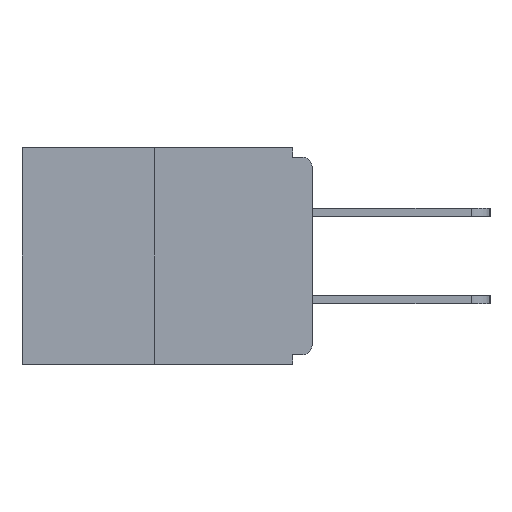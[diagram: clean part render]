
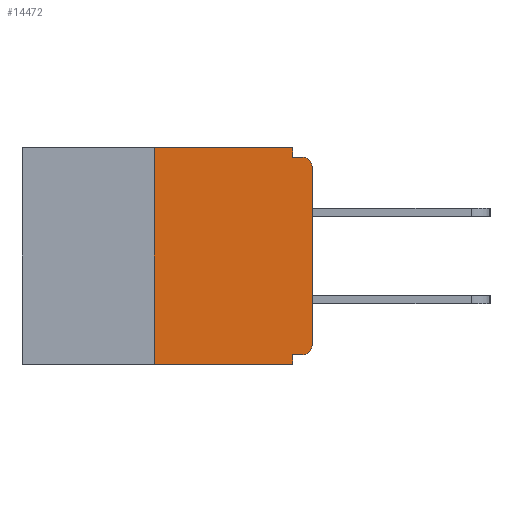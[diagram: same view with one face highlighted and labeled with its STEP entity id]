
A CAD part, left-side view. The second image highlights one B-rep face of the part: STEP entity #14472.
In plain terms, the highlighted planar face has unit normal (-1, 0, 0).
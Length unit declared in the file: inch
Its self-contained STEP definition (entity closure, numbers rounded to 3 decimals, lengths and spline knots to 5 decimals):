
#118 = CARTESIAN_POINT ( 'NONE',  ( 0., 0.031, -0.015 ) ) ;
#209 = EDGE_LOOP ( 'NONE', ( #5917, #5227, #5291, #6892, #12937, #18558, #6004, #6676, #10286, #1677 ) ) ;
#473 = LINE ( 'NONE', #4904, #12298 ) ;
#1065 = LINE ( 'NONE', #17135, #3573 ) ;
#1113 = VERTEX_POINT ( 'NONE', #13116 ) ;
#1170 = VERTEX_POINT ( 'NONE', #118 ) ;
#1677 = ORIENTED_EDGE ( 'NONE', *, *, #4137, .F. ) ;
#2107 = VECTOR ( 'NONE', #5699, 39.37008 ) ;
#2687 = LINE ( 'NONE', #16053, #6872 ) ;
#2842 = EDGE_CURVE ( 'NONE', #9294, #6440, #13365, .T. ) ;
#2954 = VECTOR ( 'NONE', #10783, 39.37008 ) ;
#3323 = DIRECTION ( 'NONE',  ( 0., 0., -1. ) ) ;
#3372 = FACE_OUTER_BOUND ( 'NONE', #209, .T. ) ;
#3427 = CARTESIAN_POINT ( 'NONE',  ( 0., 0.25, 0. ) ) ;
#3495 = LINE ( 'NONE', #5316, #2107 ) ;
#3540 = DIRECTION ( 'NONE',  ( 0., -1., 0. ) ) ;
#3573 = VECTOR ( 'NONE', #3954, 39.37008 ) ;
#3954 = DIRECTION ( 'NONE',  ( 0., 0., 1. ) ) ;
#4137 = EDGE_CURVE ( 'NONE', #6933, #1170, #2687, .T. ) ;
#4348 = CARTESIAN_POINT ( 'NONE',  ( 0., 0., -0.313 ) ) ;
#4477 = EDGE_CURVE ( 'NONE', #4915, #15543, #11458, .T. ) ;
#4904 = CARTESIAN_POINT ( 'NONE',  ( 0., 0., -0.015 ) ) ;
#4915 = VERTEX_POINT ( 'NONE', #7702 ) ;
#5026 = LINE ( 'NONE', #6744, #2954 ) ;
#5061 = AXIS2_PLACEMENT_3D ( 'NONE', #12274, #10726, #3323 ) ;
#5227 = ORIENTED_EDGE ( 'NONE', *, *, #18360, .F. ) ;
#5260 = EDGE_CURVE ( 'NONE', #12214, #6933, #15284, .T. ) ;
#5291 = ORIENTED_EDGE ( 'NONE', *, *, #8404, .T. ) ;
#5316 = CARTESIAN_POINT ( 'NONE',  ( 0., 0.031, -0.343 ) ) ;
#5699 = DIRECTION ( 'NONE',  ( 0., 0., -1. ) ) ;
#5917 = ORIENTED_EDGE ( 'NONE', *, *, #5260, .F. ) ;
#6004 = ORIENTED_EDGE ( 'NONE', *, *, #16508, .T. ) ;
#6143 = EDGE_CURVE ( 'NONE', #13521, #8086, #3495, .T. ) ;
#6440 = VERTEX_POINT ( 'NONE', #4348 ) ;
#6529 = PLANE ( 'NONE',  #10798 ) ;
#6571 = CARTESIAN_POINT ( 'NONE',  ( 0., 0.031, -0.328 ) ) ;
#6676 = ORIENTED_EDGE ( 'NONE', *, *, #4477, .T. ) ;
#6744 = CARTESIAN_POINT ( 'NONE',  ( 0., 0.46, -0.343 ) ) ;
#6872 = VECTOR ( 'NONE', #14430, 39.37008 ) ;
#6892 = ORIENTED_EDGE ( 'NONE', *, *, #6143, .F. ) ;
#6933 = VERTEX_POINT ( 'NONE', #13728 ) ;
#6989 = DIRECTION ( 'NONE',  ( -1., 0., 0. ) ) ;
#7557 = EDGE_CURVE ( 'NONE', #1170, #15543, #473, .T. ) ;
#7702 = CARTESIAN_POINT ( 'NONE',  ( 0., 0., -0.03 ) ) ;
#8086 = VERTEX_POINT ( 'NONE', #16909 ) ;
#8404 = EDGE_CURVE ( 'NONE', #1113, #8086, #5026, .T. ) ;
#9294 = VERTEX_POINT ( 'NONE', #12240 ) ;
#9694 = CARTESIAN_POINT ( 'NONE',  ( 0., 0.46, 0. ) ) ;
#10286 = ORIENTED_EDGE ( 'NONE', *, *, #7557, .F. ) ;
#10726 = DIRECTION ( 'NONE',  ( -1., 0., 0. ) ) ;
#10783 = DIRECTION ( 'NONE',  ( 0., -1., 0. ) ) ;
#10798 = AXIS2_PLACEMENT_3D ( 'NONE', #18547, #14040, #12685 ) ;
#11179 = CARTESIAN_POINT ( 'NONE',  ( 0., 0., -0.328 ) ) ;
#11458 = CIRCLE ( 'NONE', #18222, 0.015 ) ;
#12096 = CARTESIAN_POINT ( 'NONE',  ( 0., 0.015, -0.015 ) ) ;
#12213 = DIRECTION ( 'NONE',  ( 0., -1., 0. ) ) ;
#12214 = VERTEX_POINT ( 'NONE', #3427 ) ;
#12240 = CARTESIAN_POINT ( 'NONE',  ( 0., 0.015, -0.328 ) ) ;
#12274 = CARTESIAN_POINT ( 'NONE',  ( 0., 0.015, -0.313 ) ) ;
#12298 = VECTOR ( 'NONE', #12213, 39.37008 ) ;
#12685 = DIRECTION ( 'NONE',  ( 0., 0., -1. ) ) ;
#12698 = EDGE_CURVE ( 'NONE', #9294, #13521, #15523, .T. ) ;
#12937 = ORIENTED_EDGE ( 'NONE', *, *, #12698, .F. ) ;
#13116 = CARTESIAN_POINT ( 'NONE',  ( 0., 0.25, -0.343 ) ) ;
#13365 = CIRCLE ( 'NONE', #5061, 0.015 ) ;
#13521 = VERTEX_POINT ( 'NONE', #6571 ) ;
#13600 = CARTESIAN_POINT ( 'NONE',  ( 0., 0., 0. ) ) ;
#13697 = DIRECTION ( 'NONE',  ( 0., 0., 1. ) ) ;
#13728 = CARTESIAN_POINT ( 'NONE',  ( 0., 0.031, 0. ) ) ;
#13776 = VECTOR ( 'NONE', #18589, 39.37008 ) ;
#14040 = DIRECTION ( 'NONE',  ( 1., 0., 0. ) ) ;
#14406 = DIRECTION ( 'NONE',  ( 0., 0., -1. ) ) ;
#14430 = DIRECTION ( 'NONE',  ( 0., 0., -1. ) ) ;
#14472 = ADVANCED_FACE ( 'NONE', ( #3372 ), #6529, .F. ) ;
#15230 = LINE ( 'NONE', #13600, #15799 ) ;
#15284 = LINE ( 'NONE', #9694, #18989 ) ;
#15523 = LINE ( 'NONE', #11179, #13776 ) ;
#15543 = VERTEX_POINT ( 'NONE', #12096 ) ;
#15799 = VECTOR ( 'NONE', #13697, 39.37008 ) ;
#16033 = CARTESIAN_POINT ( 'NONE',  ( 0., 0.015, -0.03 ) ) ;
#16053 = CARTESIAN_POINT ( 'NONE',  ( 0., 0.031, 0. ) ) ;
#16508 = EDGE_CURVE ( 'NONE', #6440, #4915, #15230, .T. ) ;
#16909 = CARTESIAN_POINT ( 'NONE',  ( 0., 0.031, -0.343 ) ) ;
#17135 = CARTESIAN_POINT ( 'NONE',  ( 0., 0.25, 0. ) ) ;
#18222 = AXIS2_PLACEMENT_3D ( 'NONE', #16033, #6989, #14406 ) ;
#18360 = EDGE_CURVE ( 'NONE', #1113, #12214, #1065, .T. ) ;
#18547 = CARTESIAN_POINT ( 'NONE',  ( 0., 0.46, 0. ) ) ;
#18558 = ORIENTED_EDGE ( 'NONE', *, *, #2842, .T. ) ;
#18589 = DIRECTION ( 'NONE',  ( 0., 1., 0. ) ) ;
#18989 = VECTOR ( 'NONE', #3540, 39.37008 ) ;
